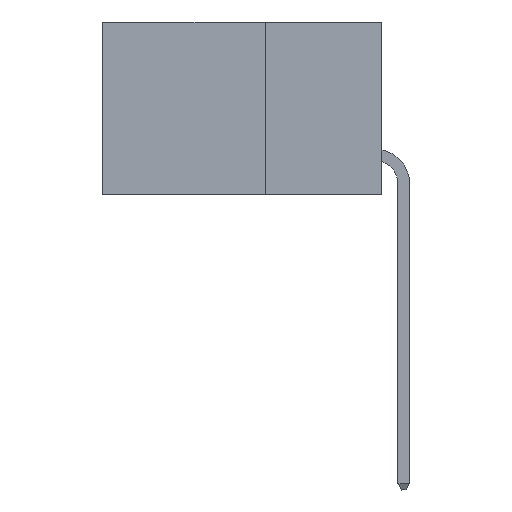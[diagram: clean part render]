
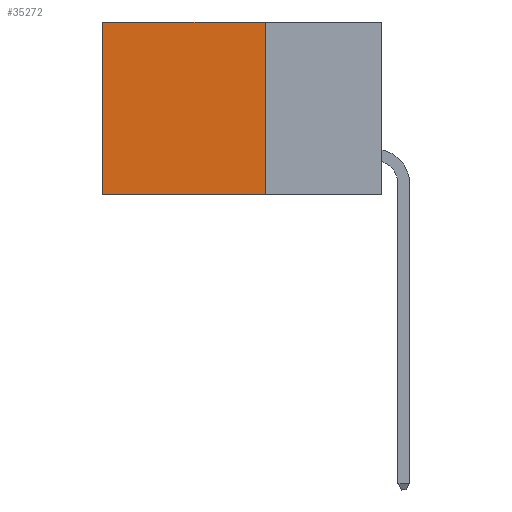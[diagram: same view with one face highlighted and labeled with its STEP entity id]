
A CAD part, left-side view. The second image highlights one B-rep face of the part: STEP entity #35272.
In plain terms, the highlighted planar face has unit normal (-1, 0, 0).
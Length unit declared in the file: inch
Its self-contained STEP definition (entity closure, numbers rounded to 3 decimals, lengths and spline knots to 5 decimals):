
#1294 = CARTESIAN_POINT ( 'NONE',  ( 0.2875, 0.25, 0. ) ) ;
#1760 = EDGE_LOOP ( 'NONE', ( #38352, #29434, #11309, #23874 ) ) ;
#2401 = DIRECTION ( 'NONE',  ( 0., 0., -1. ) ) ;
#3524 = DIRECTION ( 'NONE',  ( 0., 1., 0. ) ) ;
#6071 = CARTESIAN_POINT ( 'NONE',  ( 0.2875, 0.6, -0.37 ) ) ;
#7166 = VERTEX_POINT ( 'NONE', #42610 ) ;
#7198 = EDGE_CURVE ( 'NONE', #7166, #39405, #13087, .T. ) ;
#8439 = EDGE_CURVE ( 'NONE', #7166, #36532, #36069, .T. ) ;
#11309 = ORIENTED_EDGE ( 'NONE', *, *, #7198, .F. ) ;
#13087 = LINE ( 'NONE', #32835, #32004 ) ;
#14628 = DIRECTION ( 'NONE',  ( 0., 0., -1. ) ) ;
#15919 = CARTESIAN_POINT ( 'NONE',  ( 0.2875, 0.25, -0.37 ) ) ;
#17639 = DIRECTION ( 'NONE',  ( 0., 1., 0. ) ) ;
#18685 = CARTESIAN_POINT ( 'NONE',  ( 0.2875, 0.6, 0. ) ) ;
#20064 = CARTESIAN_POINT ( 'NONE',  ( 0.2875, 0.25, -0.37 ) ) ;
#21524 = CARTESIAN_POINT ( 'NONE',  ( 0.2875, 0.6, 0. ) ) ;
#22434 = EDGE_CURVE ( 'NONE', #39405, #34757, #42922, .T. ) ;
#23874 = ORIENTED_EDGE ( 'NONE', *, *, #8439, .T. ) ;
#26246 = DIRECTION ( 'NONE',  ( 0., 0., -1. ) ) ;
#26564 = VECTOR ( 'NONE', #14628, 39.37008 ) ;
#28593 = FACE_OUTER_BOUND ( 'NONE', #1760, .T. ) ;
#28759 = CARTESIAN_POINT ( 'NONE',  ( 0.2875, 0.25, 0. ) ) ;
#29434 = ORIENTED_EDGE ( 'NONE', *, *, #22434, .F. ) ;
#32004 = VECTOR ( 'NONE', #26246, 39.37008 ) ;
#32368 = LINE ( 'NONE', #21524, #26564 ) ;
#32835 = CARTESIAN_POINT ( 'NONE',  ( 0.2875, 0.25, 0. ) ) ;
#32905 = VECTOR ( 'NONE', #17639, 39.37008 ) ;
#32941 = VECTOR ( 'NONE', #3524, 39.37008 ) ;
#34757 = VERTEX_POINT ( 'NONE', #6071 ) ;
#35272 = ADVANCED_FACE ( 'NONE', ( #28593 ), #38596, .F. ) ;
#35345 = DIRECTION ( 'NONE',  ( 1., 0., 0. ) ) ;
#36069 = LINE ( 'NONE', #1294, #32905 ) ;
#36532 = VERTEX_POINT ( 'NONE', #18685 ) ;
#38352 = ORIENTED_EDGE ( 'NONE', *, *, #42900, .T. ) ;
#38588 = AXIS2_PLACEMENT_3D ( 'NONE', #28759, #35345, #2401 ) ;
#38596 = PLANE ( 'NONE',  #38588 ) ;
#39405 = VERTEX_POINT ( 'NONE', #15919 ) ;
#42610 = CARTESIAN_POINT ( 'NONE',  ( 0.2875, 0.25, 0. ) ) ;
#42900 = EDGE_CURVE ( 'NONE', #36532, #34757, #32368, .T. ) ;
#42922 = LINE ( 'NONE', #20064, #32941 ) ;
